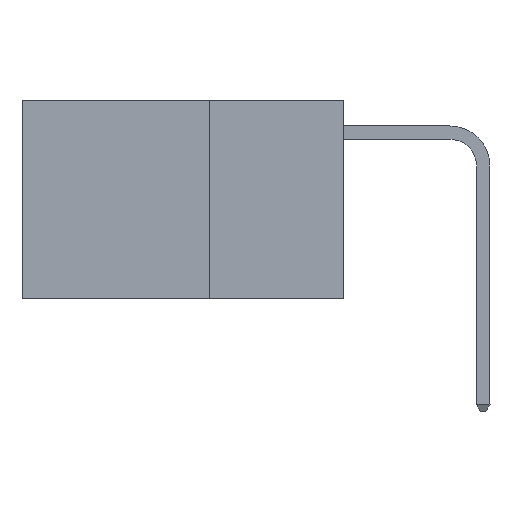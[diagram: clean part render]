
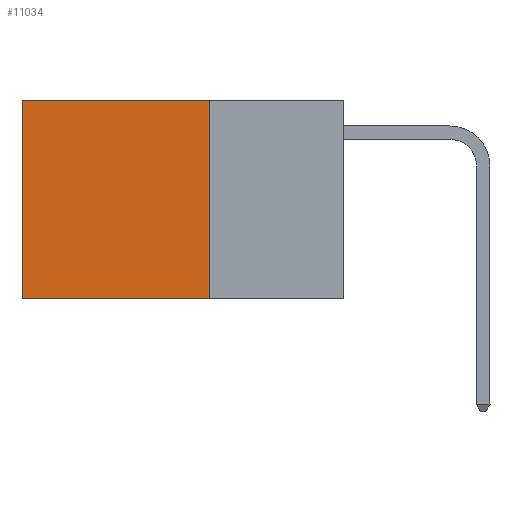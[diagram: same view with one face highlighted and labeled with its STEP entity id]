
A CAD part, left-side view. The second image highlights one B-rep face of the part: STEP entity #11034.
In plain terms, the highlighted planar face has unit normal (-1, 0, 0).
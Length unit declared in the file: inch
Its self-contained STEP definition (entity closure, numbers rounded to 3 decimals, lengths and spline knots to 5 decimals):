
#1709 = DIRECTION ( 'NONE',  ( 0., 0., -1. ) ) ;
#3011 = VECTOR ( 'NONE', #1709, 39.37008 ) ;
#3328 = DIRECTION ( 'NONE',  ( 0., 1., 0. ) ) ;
#3535 = LINE ( 'NONE', #17093, #3011 ) ;
#3965 = CARTESIAN_POINT ( 'NONE',  ( 0.2625, 0.6, -0.37 ) ) ;
#4874 = VERTEX_POINT ( 'NONE', #3965 ) ;
#5728 = DIRECTION ( 'NONE',  ( 0., 1., 0. ) ) ;
#6619 = DIRECTION ( 'NONE',  ( 1., 0., 0. ) ) ;
#7270 = CARTESIAN_POINT ( 'NONE',  ( 0.2625, 0.25, 0. ) ) ;
#7558 = EDGE_CURVE ( 'NONE', #13392, #4874, #15685, .T. ) ;
#8000 = FACE_OUTER_BOUND ( 'NONE', #9519, .T. ) ;
#8992 = ORIENTED_EDGE ( 'NONE', *, *, #7558, .F. ) ;
#9244 = CARTESIAN_POINT ( 'NONE',  ( 0.2625, 0.25, 0. ) ) ;
#9519 = EDGE_LOOP ( 'NONE', ( #19742, #8992, #15082, #11266 ) ) ;
#9592 = VERTEX_POINT ( 'NONE', #7270 ) ;
#9912 = EDGE_CURVE ( 'NONE', #17774, #4874, #3535, .T. ) ;
#10029 = VECTOR ( 'NONE', #5728, 39.37008 ) ;
#10130 = AXIS2_PLACEMENT_3D ( 'NONE', #16895, #6619, #18655 ) ;
#11034 = ADVANCED_FACE ( 'NONE', ( #8000 ), #16823, .F. ) ;
#11107 = LINE ( 'NONE', #9244, #20313 ) ;
#11266 = ORIENTED_EDGE ( 'NONE', *, *, #19176, .T. ) ;
#13392 = VERTEX_POINT ( 'NONE', #15178 ) ;
#14367 = DIRECTION ( 'NONE',  ( 0., 0., -1. ) ) ;
#15082 = ORIENTED_EDGE ( 'NONE', *, *, #18491, .F. ) ;
#15178 = CARTESIAN_POINT ( 'NONE',  ( 0.2625, 0.25, -0.37 ) ) ;
#15685 = LINE ( 'NONE', #22146, #20293 ) ;
#16028 = CARTESIAN_POINT ( 'NONE',  ( 0.2625, 0.25, 0. ) ) ;
#16823 = PLANE ( 'NONE',  #10130 ) ;
#16895 = CARTESIAN_POINT ( 'NONE',  ( 0.2625, 0.25, 0. ) ) ;
#17093 = CARTESIAN_POINT ( 'NONE',  ( 0.2625, 0.6, 0. ) ) ;
#17774 = VERTEX_POINT ( 'NONE', #19144 ) ;
#18491 = EDGE_CURVE ( 'NONE', #9592, #13392, #11107, .T. ) ;
#18655 = DIRECTION ( 'NONE',  ( 0., 0., -1. ) ) ;
#19144 = CARTESIAN_POINT ( 'NONE',  ( 0.2625, 0.6, 0. ) ) ;
#19176 = EDGE_CURVE ( 'NONE', #9592, #17774, #19228, .T. ) ;
#19228 = LINE ( 'NONE', #16028, #10029 ) ;
#19742 = ORIENTED_EDGE ( 'NONE', *, *, #9912, .T. ) ;
#20293 = VECTOR ( 'NONE', #3328, 39.37008 ) ;
#20313 = VECTOR ( 'NONE', #14367, 39.37008 ) ;
#22146 = CARTESIAN_POINT ( 'NONE',  ( 0.2625, 0.25, -0.37 ) ) ;
